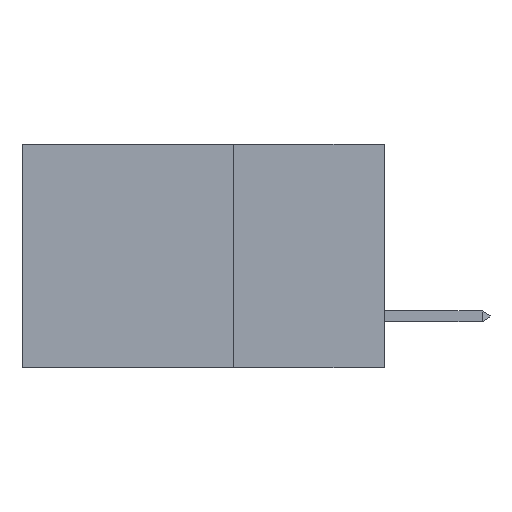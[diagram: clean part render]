
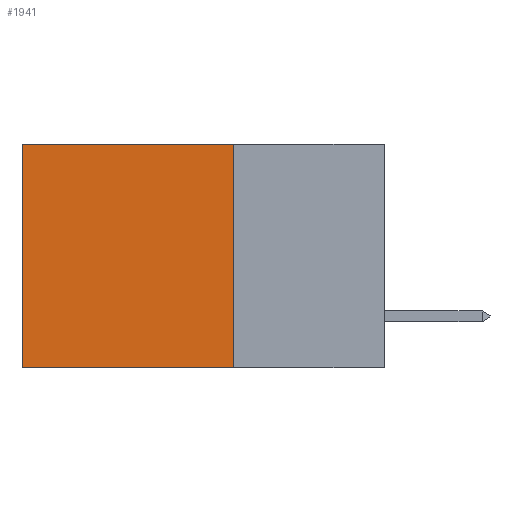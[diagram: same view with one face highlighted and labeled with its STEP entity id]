
A CAD part, left-side view. The second image highlights one B-rep face of the part: STEP entity #1941.
In plain terms, the highlighted planar face has unit normal (-1, 0, 0).
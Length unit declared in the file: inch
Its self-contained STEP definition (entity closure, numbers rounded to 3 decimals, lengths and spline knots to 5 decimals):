
#373 = VECTOR ( 'NONE', #2801, 39.37008 ) ;
#586 = DIRECTION ( 'NONE',  ( 0., 0., -1. ) ) ;
#692 = CARTESIAN_POINT ( 'NONE',  ( 0.2875, 0.6, 0. ) ) ;
#1134 = VECTOR ( 'NONE', #10012, 39.37008 ) ;
#1305 = ORIENTED_EDGE ( 'NONE', *, *, #5464, .T. ) ;
#1393 = EDGE_CURVE ( 'NONE', #16143, #9636, #16357, .T. ) ;
#1608 = CARTESIAN_POINT ( 'NONE',  ( 0.2875, 0.6, 0. ) ) ;
#1763 = CARTESIAN_POINT ( 'NONE',  ( 0.2875, 0.25, 0. ) ) ;
#1941 = ADVANCED_FACE ( 'NONE', ( #14690 ), #10835, .F. ) ;
#2256 = ORIENTED_EDGE ( 'NONE', *, *, #3340, .T. ) ;
#2801 = DIRECTION ( 'NONE',  ( 0., 0., -1. ) ) ;
#2981 = CARTESIAN_POINT ( 'NONE',  ( 0.2875, 0.25, 0. ) ) ;
#3340 = EDGE_CURVE ( 'NONE', #10015, #8247, #8778, .T. ) ;
#3977 = EDGE_CURVE ( 'NONE', #10015, #16143, #5611, .T. ) ;
#5464 = EDGE_CURVE ( 'NONE', #8247, #9636, #7317, .T. ) ;
#5608 = ORIENTED_EDGE ( 'NONE', *, *, #1393, .F. ) ;
#5611 = LINE ( 'NONE', #2981, #373 ) ;
#5828 = DIRECTION ( 'NONE',  ( 1., 0., 0. ) ) ;
#7317 = LINE ( 'NONE', #692, #1134 ) ;
#7367 = VECTOR ( 'NONE', #16283, 39.37008 ) ;
#8210 = EDGE_LOOP ( 'NONE', ( #1305, #5608, #9904, #2256 ) ) ;
#8247 = VERTEX_POINT ( 'NONE', #1608 ) ;
#8606 = VECTOR ( 'NONE', #8695, 39.37008 ) ;
#8695 = DIRECTION ( 'NONE',  ( 0., 1., 0. ) ) ;
#8778 = LINE ( 'NONE', #11405, #7367 ) ;
#8857 = AXIS2_PLACEMENT_3D ( 'NONE', #1763, #5828, #586 ) ;
#9636 = VERTEX_POINT ( 'NONE', #12019 ) ;
#9904 = ORIENTED_EDGE ( 'NONE', *, *, #3977, .F. ) ;
#10012 = DIRECTION ( 'NONE',  ( 0., 0., -1. ) ) ;
#10015 = VERTEX_POINT ( 'NONE', #14263 ) ;
#10669 = CARTESIAN_POINT ( 'NONE',  ( 0.2875, 0.25, -0.37 ) ) ;
#10835 = PLANE ( 'NONE',  #8857 ) ;
#11400 = CARTESIAN_POINT ( 'NONE',  ( 0.2875, 0.25, -0.37 ) ) ;
#11405 = CARTESIAN_POINT ( 'NONE',  ( 0.2875, 0.25, 0. ) ) ;
#12019 = CARTESIAN_POINT ( 'NONE',  ( 0.2875, 0.6, -0.37 ) ) ;
#14263 = CARTESIAN_POINT ( 'NONE',  ( 0.2875, 0.25, 0. ) ) ;
#14690 = FACE_OUTER_BOUND ( 'NONE', #8210, .T. ) ;
#16143 = VERTEX_POINT ( 'NONE', #10669 ) ;
#16283 = DIRECTION ( 'NONE',  ( 0., 1., 0. ) ) ;
#16357 = LINE ( 'NONE', #11400, #8606 ) ;
